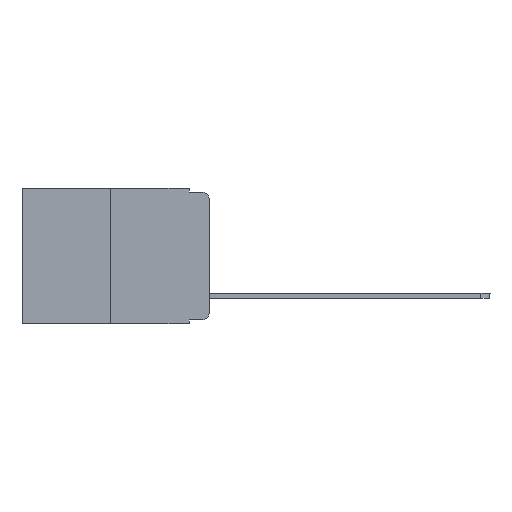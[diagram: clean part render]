
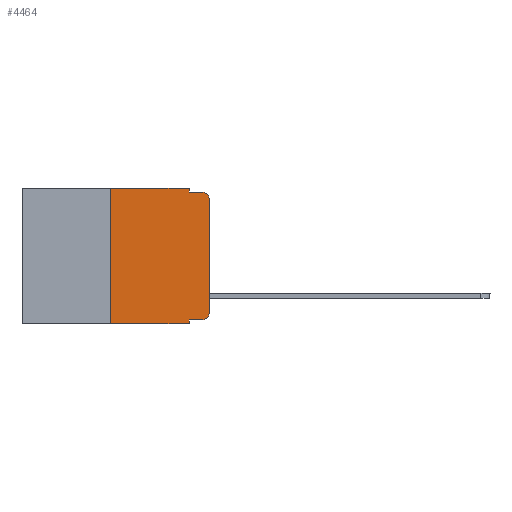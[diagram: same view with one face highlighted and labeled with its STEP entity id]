
A CAD part, left-side view. The second image highlights one B-rep face of the part: STEP entity #4464.
In plain terms, the highlighted planar face has unit normal (-1, 0, 0).
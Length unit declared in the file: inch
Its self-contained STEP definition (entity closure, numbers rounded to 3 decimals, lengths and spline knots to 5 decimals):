
#82 = EDGE_CURVE ( 'NONE', #2173, #5742, #2877, .T. ) ;
#315 = CARTESIAN_POINT ( 'NONE',  ( 0., 0.051, 0. ) ) ;
#416 = DIRECTION ( 'NONE',  ( 0., 0., -1. ) ) ;
#495 = DIRECTION ( 'NONE',  ( 0., 0., -1. ) ) ;
#512 = CARTESIAN_POINT ( 'NONE',  ( 0., 0.051, -0.01 ) ) ;
#790 = CARTESIAN_POINT ( 'NONE',  ( 0., 0., -0.313 ) ) ;
#801 = AXIS2_PLACEMENT_3D ( 'NONE', #6508, #7335, #7227 ) ;
#977 = CARTESIAN_POINT ( 'NONE',  ( 0., 0.051, -0.01 ) ) ;
#1013 = EDGE_LOOP ( 'NONE', ( #6070, #6423, #2552, #5384, #8083, #6916, #3860, #1093, #4364, #4110 ) ) ;
#1093 = ORIENTED_EDGE ( 'NONE', *, *, #9503, .F. ) ;
#1171 = CARTESIAN_POINT ( 'NONE',  ( 0., 0.473, 0. ) ) ;
#1506 = CARTESIAN_POINT ( 'NONE',  ( 0., 0.051, 0. ) ) ;
#1813 = CARTESIAN_POINT ( 'NONE',  ( 0., 0.25, -0.343 ) ) ;
#1996 = CARTESIAN_POINT ( 'NONE',  ( 0., 0.051, 0. ) ) ;
#2066 = DIRECTION ( 'NONE',  ( 0., -1., 0. ) ) ;
#2173 = VERTEX_POINT ( 'NONE', #512 ) ;
#2552 = ORIENTED_EDGE ( 'NONE', *, *, #82, .F. ) ;
#2877 = LINE ( 'NONE', #977, #2975 ) ;
#2903 = LINE ( 'NONE', #1996, #4562 ) ;
#2913 = VERTEX_POINT ( 'NONE', #315 ) ;
#2925 = EDGE_CURVE ( 'NONE', #5535, #2913, #8210, .T. ) ;
#2975 = VECTOR ( 'NONE', #6082, 39.37008 ) ;
#2988 = EDGE_CURVE ( 'NONE', #5356, #5742, #9884, .T. ) ;
#3318 = EDGE_CURVE ( 'NONE', #2913, #2173, #2903, .T. ) ;
#3509 = DIRECTION ( 'NONE',  ( 0., 0., 1. ) ) ;
#3624 = PLANE ( 'NONE',  #9236 ) ;
#3829 = EDGE_CURVE ( 'NONE', #9965, #5535, #10935, .T. ) ;
#3860 = ORIENTED_EDGE ( 'NONE', *, *, #6345, .T. ) ;
#4032 = VECTOR ( 'NONE', #10031, 39.37008 ) ;
#4110 = ORIENTED_EDGE ( 'NONE', *, *, #10616, .T. ) ;
#4156 = CARTESIAN_POINT ( 'NONE',  ( 0., 0.25, 0. ) ) ;
#4259 = CARTESIAN_POINT ( 'NONE',  ( 0., 0.25, 0. ) ) ;
#4302 = CARTESIAN_POINT ( 'NONE',  ( 0., 0., 0. ) ) ;
#4364 = ORIENTED_EDGE ( 'NONE', *, *, #5026, .T. ) ;
#4464 = ADVANCED_FACE ( 'NONE', ( #7872 ), #3624, .F. ) ;
#4562 = VECTOR ( 'NONE', #6321, 39.37008 ) ;
#4652 = VECTOR ( 'NONE', #3509, 39.37008 ) ;
#4685 = CARTESIAN_POINT ( 'NONE',  ( 0., 0.051, -0.343 ) ) ;
#4735 = LINE ( 'NONE', #8127, #8559 ) ;
#4835 = EDGE_CURVE ( 'NONE', #7724, #5356, #10402, .T. ) ;
#5026 = EDGE_CURVE ( 'NONE', #9417, #5994, #4735, .T. ) ;
#5091 = VECTOR ( 'NONE', #2066, 39.37008 ) ;
#5356 = VERTEX_POINT ( 'NONE', #5628 ) ;
#5384 = ORIENTED_EDGE ( 'NONE', *, *, #3318, .F. ) ;
#5535 = VERTEX_POINT ( 'NONE', #4259 ) ;
#5559 = DIRECTION ( 'NONE',  ( -1., 0., 0. ) ) ;
#5628 = CARTESIAN_POINT ( 'NONE',  ( 0., 0., -0.03 ) ) ;
#5742 = VERTEX_POINT ( 'NONE', #10285 ) ;
#5994 = VERTEX_POINT ( 'NONE', #9613 ) ;
#6070 = ORIENTED_EDGE ( 'NONE', *, *, #4835, .T. ) ;
#6082 = DIRECTION ( 'NONE',  ( 0., -1., 0. ) ) ;
#6231 = AXIS2_PLACEMENT_3D ( 'NONE', #6681, #5559, #495 ) ;
#6321 = DIRECTION ( 'NONE',  ( 0., 0., -1. ) ) ;
#6345 = EDGE_CURVE ( 'NONE', #9965, #6614, #9242, .T. ) ;
#6416 = CIRCLE ( 'NONE', #6231, 0.02 ) ;
#6423 = ORIENTED_EDGE ( 'NONE', *, *, #2988, .T. ) ;
#6486 = DIRECTION ( 'NONE',  ( 0., -1., 0. ) ) ;
#6508 = CARTESIAN_POINT ( 'NONE',  ( 0., 0.02, -0.03 ) ) ;
#6614 = VERTEX_POINT ( 'NONE', #4685 ) ;
#6681 = CARTESIAN_POINT ( 'NONE',  ( 0., 0.02, -0.313 ) ) ;
#6890 = DIRECTION ( 'NONE',  ( 0., -1., 0. ) ) ;
#6916 = ORIENTED_EDGE ( 'NONE', *, *, #3829, .F. ) ;
#7054 = CARTESIAN_POINT ( 'NONE',  ( 0., 0.473, 0. ) ) ;
#7227 = DIRECTION ( 'NONE',  ( 0., 0., -1. ) ) ;
#7335 = DIRECTION ( 'NONE',  ( -1., 0., 0. ) ) ;
#7724 = VERTEX_POINT ( 'NONE', #790 ) ;
#7872 = FACE_OUTER_BOUND ( 'NONE', #1013, .T. ) ;
#8029 = DIRECTION ( 'NONE',  ( 1., 0., 0. ) ) ;
#8083 = ORIENTED_EDGE ( 'NONE', *, *, #2925, .F. ) ;
#8127 = CARTESIAN_POINT ( 'NONE',  ( 0., 0.051, -0.333 ) ) ;
#8154 = CARTESIAN_POINT ( 'NONE',  ( 0., 0.051, -0.333 ) ) ;
#8210 = LINE ( 'NONE', #1171, #5091 ) ;
#8559 = VECTOR ( 'NONE', #6486, 39.37008 ) ;
#9207 = DIRECTION ( 'NONE',  ( 0., 0., 1. ) ) ;
#9236 = AXIS2_PLACEMENT_3D ( 'NONE', #7054, #8029, #416 ) ;
#9242 = LINE ( 'NONE', #9296, #9529 ) ;
#9296 = CARTESIAN_POINT ( 'NONE',  ( 0., 0.473, -0.343 ) ) ;
#9417 = VERTEX_POINT ( 'NONE', #8154 ) ;
#9503 = EDGE_CURVE ( 'NONE', #9417, #6614, #9925, .T. ) ;
#9529 = VECTOR ( 'NONE', #6890, 39.37008 ) ;
#9613 = CARTESIAN_POINT ( 'NONE',  ( 0., 0.02, -0.333 ) ) ;
#9884 = CIRCLE ( 'NONE', #801, 0.02 ) ;
#9925 = LINE ( 'NONE', #1506, #4032 ) ;
#9965 = VERTEX_POINT ( 'NONE', #1813 ) ;
#10031 = DIRECTION ( 'NONE',  ( 0., 0., -1. ) ) ;
#10285 = CARTESIAN_POINT ( 'NONE',  ( 0., 0.02, -0.01 ) ) ;
#10402 = LINE ( 'NONE', #4302, #4652 ) ;
#10616 = EDGE_CURVE ( 'NONE', #5994, #7724, #6416, .T. ) ;
#10774 = VECTOR ( 'NONE', #9207, 39.37008 ) ;
#10935 = LINE ( 'NONE', #4156, #10774 ) ;
